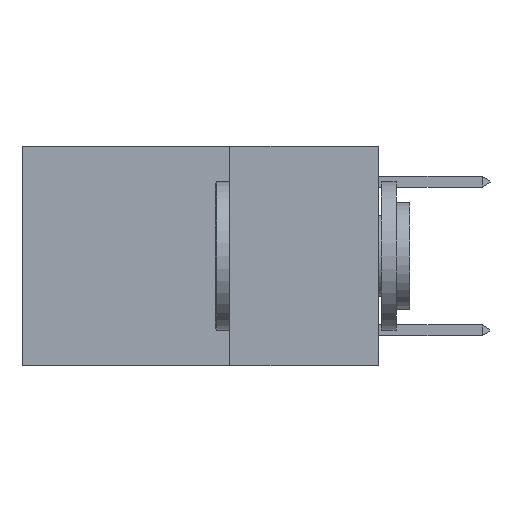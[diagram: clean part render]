
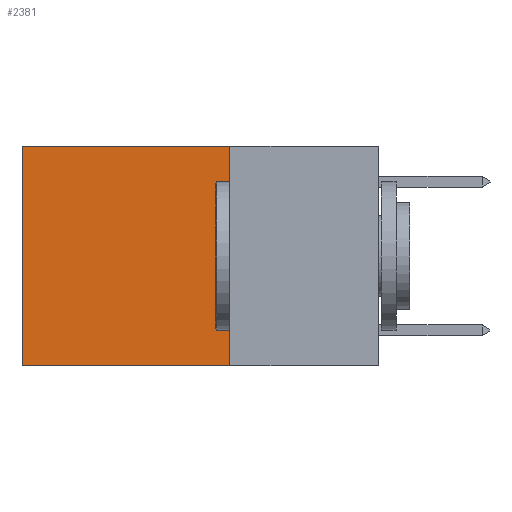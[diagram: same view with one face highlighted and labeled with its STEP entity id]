
A CAD part, left-side view. The second image highlights one B-rep face of the part: STEP entity #2381.
In plain terms, the highlighted planar face has unit normal (-1, 0, 0).
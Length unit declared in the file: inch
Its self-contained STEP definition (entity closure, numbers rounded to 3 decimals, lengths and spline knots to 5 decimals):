
#846 = ORIENTED_EDGE ( 'NONE', *, *, #16259, .F. ) ;
#1568 = VECTOR ( 'NONE', #1580, 39.37008 ) ;
#1580 = DIRECTION ( 'NONE',  ( 0., 1., 0. ) ) ;
#2381 = ADVANCED_FACE ( 'NONE', ( #4813 ), #7539, .F. ) ;
#2388 = CARTESIAN_POINT ( 'NONE',  ( 0.2625, 0.6, -0.37 ) ) ;
#2528 = EDGE_LOOP ( 'NONE', ( #18743, #3379, #846, #3711 ) ) ;
#2724 = VERTEX_POINT ( 'NONE', #14230 ) ;
#3379 = ORIENTED_EDGE ( 'NONE', *, *, #10466, .F. ) ;
#3412 = CARTESIAN_POINT ( 'NONE',  ( 0.2625, 0.25, 0. ) ) ;
#3455 = VECTOR ( 'NONE', #5215, 39.37008 ) ;
#3711 = ORIENTED_EDGE ( 'NONE', *, *, #12458, .T. ) ;
#4266 = CARTESIAN_POINT ( 'NONE',  ( 0.2625, 0.25, -0.37 ) ) ;
#4813 = FACE_OUTER_BOUND ( 'NONE', #2528, .T. ) ;
#5121 = CARTESIAN_POINT ( 'NONE',  ( 0.2625, 0.6, 0. ) ) ;
#5215 = DIRECTION ( 'NONE',  ( 0., 0., -1. ) ) ;
#6253 = DIRECTION ( 'NONE',  ( 0., 1., 0. ) ) ;
#6480 = VECTOR ( 'NONE', #6253, 39.37008 ) ;
#7224 = VECTOR ( 'NONE', #16510, 39.37008 ) ;
#7539 = PLANE ( 'NONE',  #13664 ) ;
#7715 = LINE ( 'NONE', #3412, #6480 ) ;
#7856 = LINE ( 'NONE', #5121, #3455 ) ;
#7946 = LINE ( 'NONE', #8996, #1568 ) ;
#8996 = CARTESIAN_POINT ( 'NONE',  ( 0.2625, 0.25, -0.37 ) ) ;
#10466 = EDGE_CURVE ( 'NONE', #16614, #11795, #7946, .T. ) ;
#10759 = CARTESIAN_POINT ( 'NONE',  ( 0.2625, 0.25, 0. ) ) ;
#11795 = VERTEX_POINT ( 'NONE', #2388 ) ;
#12458 = EDGE_CURVE ( 'NONE', #2724, #17344, #7715, .T. ) ;
#13664 = AXIS2_PLACEMENT_3D ( 'NONE', #10759, #15055, #15253 ) ;
#13857 = CARTESIAN_POINT ( 'NONE',  ( 0.2625, 0.25, 0. ) ) ;
#14230 = CARTESIAN_POINT ( 'NONE',  ( 0.2625, 0.25, 0. ) ) ;
#15055 = DIRECTION ( 'NONE',  ( 1., 0., 0. ) ) ;
#15253 = DIRECTION ( 'NONE',  ( 0., 0., -1. ) ) ;
#15953 = EDGE_CURVE ( 'NONE', #17344, #11795, #7856, .T. ) ;
#16259 = EDGE_CURVE ( 'NONE', #2724, #16614, #16704, .T. ) ;
#16510 = DIRECTION ( 'NONE',  ( 0., 0., -1. ) ) ;
#16614 = VERTEX_POINT ( 'NONE', #4266 ) ;
#16704 = LINE ( 'NONE', #13857, #7224 ) ;
#17344 = VERTEX_POINT ( 'NONE', #18605 ) ;
#18605 = CARTESIAN_POINT ( 'NONE',  ( 0.2625, 0.6, 0. ) ) ;
#18743 = ORIENTED_EDGE ( 'NONE', *, *, #15953, .T. ) ;
